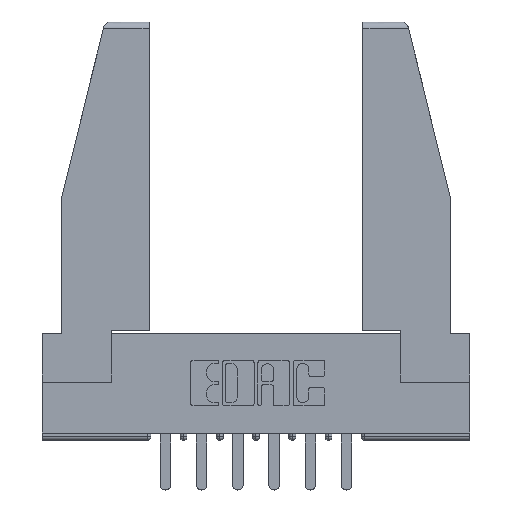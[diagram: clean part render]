
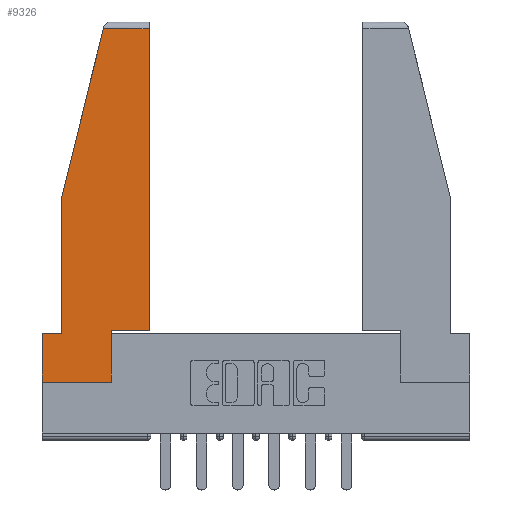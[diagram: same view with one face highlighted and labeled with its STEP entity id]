
A CAD part, top view. The second image highlights one B-rep face of the part: STEP entity #9326.
In plain terms, the highlighted planar face has unit normal (0, 0, 1).
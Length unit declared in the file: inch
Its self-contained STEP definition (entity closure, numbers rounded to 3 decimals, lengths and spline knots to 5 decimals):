
#229 = DIRECTION ( 'NONE',  ( 0., 1., 0. ) ) ;
#515 = CARTESIAN_POINT ( 'NONE',  ( 0., 0.21, 0. ) ) ;
#567 = EDGE_CURVE ( 'NONE', #11454, #3754, #2160, .T. ) ;
#851 = DIRECTION ( 'NONE',  ( 1., 0., 0. ) ) ;
#950 = VERTEX_POINT ( 'NONE', #9041 ) ;
#968 = DIRECTION ( 'NONE',  ( 1., 0., 0. ) ) ;
#1222 = VERTEX_POINT ( 'NONE', #5783 ) ;
#1435 = ORIENTED_EDGE ( 'NONE', *, *, #2425, .T. ) ;
#1486 = AXIS2_PLACEMENT_3D ( 'NONE', #10564, #9607, #851 ) ;
#1592 = VECTOR ( 'NONE', #1680, 39.37008 ) ;
#1606 = DIRECTION ( 'NONE',  ( -1., 0., 0. ) ) ;
#1680 = DIRECTION ( 'NONE',  ( -0.239, -0.971, 0. ) ) ;
#1937 = EDGE_CURVE ( 'NONE', #7378, #5546, #4932, .T. ) ;
#2131 = CARTESIAN_POINT ( 'NONE',  ( 0.297, 0.223, 0. ) ) ;
#2160 = LINE ( 'NONE', #3176, #5105 ) ;
#2229 = DIRECTION ( 'NONE',  ( 0., -1., 0. ) ) ;
#2425 = EDGE_CURVE ( 'NONE', #5546, #950, #2567, .T. ) ;
#2567 = LINE ( 'NONE', #515, #6012 ) ;
#2698 = VECTOR ( 'NONE', #2229, 39.37008 ) ;
#2805 = DIRECTION ( 'NONE',  ( 1., 0., 0. ) ) ;
#3172 = EDGE_CURVE ( 'NONE', #1222, #10334, #9831, .T. ) ;
#3176 = CARTESIAN_POINT ( 'NONE',  ( 0.297, 0., 0. ) ) ;
#3432 = EDGE_CURVE ( 'NONE', #11808, #11454, #10453, .T. ) ;
#3601 = DIRECTION ( 'NONE',  ( -1., 0., 0. ) ) ;
#3675 = FACE_OUTER_BOUND ( 'NONE', #5589, .T. ) ;
#3702 = CARTESIAN_POINT ( 'NONE',  ( 0., 0.21, 0. ) ) ;
#3754 = VERTEX_POINT ( 'NONE', #7293 ) ;
#4036 = VECTOR ( 'NONE', #229, 39.37008 ) ;
#4481 = ORIENTED_EDGE ( 'NONE', *, *, #3172, .T. ) ;
#4608 = CARTESIAN_POINT ( 'NONE',  ( 0.297, 0., 0. ) ) ;
#4710 = CARTESIAN_POINT ( 'NONE',  ( 0.271, 1.55, 0. ) ) ;
#4932 = LINE ( 'NONE', #6865, #2698 ) ;
#5105 = VECTOR ( 'NONE', #6075, 39.37008 ) ;
#5145 = CARTESIAN_POINT ( 'NONE',  ( 0.2636, 1.52, 0. ) ) ;
#5177 = CARTESIAN_POINT ( 'NONE',  ( 0.086, 0.8, 0. ) ) ;
#5462 = ORIENTED_EDGE ( 'NONE', *, *, #11203, .T. ) ;
#5466 = LINE ( 'NONE', #4710, #1592 ) ;
#5546 = VERTEX_POINT ( 'NONE', #9511 ) ;
#5555 = CARTESIAN_POINT ( 'NONE',  ( 0., 0., 0. ) ) ;
#5589 = EDGE_LOOP ( 'NONE', ( #4481, #7226, #7911, #10120, #1435, #12361, #11937, #11992, #5462 ) ) ;
#5698 = CARTESIAN_POINT ( 'NONE',  ( 0.461, 1.52, 0. ) ) ;
#5783 = CARTESIAN_POINT ( 'NONE',  ( 0.461, 0.223, 0. ) ) ;
#6012 = VECTOR ( 'NONE', #3601, 39.37008 ) ;
#6075 = DIRECTION ( 'NONE',  ( 0., 1., 0. ) ) ;
#6687 = CARTESIAN_POINT ( 'NONE',  ( 0., 1.52, 0. ) ) ;
#6865 = CARTESIAN_POINT ( 'NONE',  ( 0.086, 0.8, 0. ) ) ;
#7226 = ORIENTED_EDGE ( 'NONE', *, *, #11031, .T. ) ;
#7293 = CARTESIAN_POINT ( 'NONE',  ( 0.297, 0.223, 0. ) ) ;
#7371 = DIRECTION ( 'NONE',  ( 0., -1., 0. ) ) ;
#7375 = VECTOR ( 'NONE', #7371, 39.37008 ) ;
#7378 = VERTEX_POINT ( 'NONE', #5177 ) ;
#7828 = VERTEX_POINT ( 'NONE', #5145 ) ;
#7911 = ORIENTED_EDGE ( 'NONE', *, *, #12385, .T. ) ;
#9041 = CARTESIAN_POINT ( 'NONE',  ( 0., 0.21, 0. ) ) ;
#9069 = CARTESIAN_POINT ( 'NONE',  ( 0., 0., 0. ) ) ;
#9326 = ADVANCED_FACE ( 'NONE', ( #3675 ), #11400, .T. ) ;
#9505 = VECTOR ( 'NONE', #968, 39.37008 ) ;
#9511 = CARTESIAN_POINT ( 'NONE',  ( 0.086, 0.21, 0. ) ) ;
#9607 = DIRECTION ( 'NONE',  ( 0., 0., 1. ) ) ;
#9770 = CARTESIAN_POINT ( 'NONE',  ( 0.461, 0.223, 0. ) ) ;
#9831 = LINE ( 'NONE', #9770, #4036 ) ;
#10120 = ORIENTED_EDGE ( 'NONE', *, *, #1937, .T. ) ;
#10235 = EDGE_CURVE ( 'NONE', #950, #11808, #12410, .T. ) ;
#10334 = VERTEX_POINT ( 'NONE', #5698 ) ;
#10416 = LINE ( 'NONE', #6687, #11563 ) ;
#10453 = LINE ( 'NONE', #5555, #12011 ) ;
#10564 = CARTESIAN_POINT ( 'NONE',  ( 0., 0., 0. ) ) ;
#11031 = EDGE_CURVE ( 'NONE', #10334, #7828, #10416, .T. ) ;
#11203 = EDGE_CURVE ( 'NONE', #3754, #1222, #11907, .T. ) ;
#11400 = PLANE ( 'NONE',  #1486 ) ;
#11454 = VERTEX_POINT ( 'NONE', #4608 ) ;
#11563 = VECTOR ( 'NONE', #1606, 39.37008 ) ;
#11808 = VERTEX_POINT ( 'NONE', #9069 ) ;
#11907 = LINE ( 'NONE', #2131, #9505 ) ;
#11937 = ORIENTED_EDGE ( 'NONE', *, *, #3432, .T. ) ;
#11992 = ORIENTED_EDGE ( 'NONE', *, *, #567, .T. ) ;
#12011 = VECTOR ( 'NONE', #2805, 39.37008 ) ;
#12361 = ORIENTED_EDGE ( 'NONE', *, *, #10235, .T. ) ;
#12385 = EDGE_CURVE ( 'NONE', #7828, #7378, #5466, .T. ) ;
#12410 = LINE ( 'NONE', #3702, #7375 ) ;
